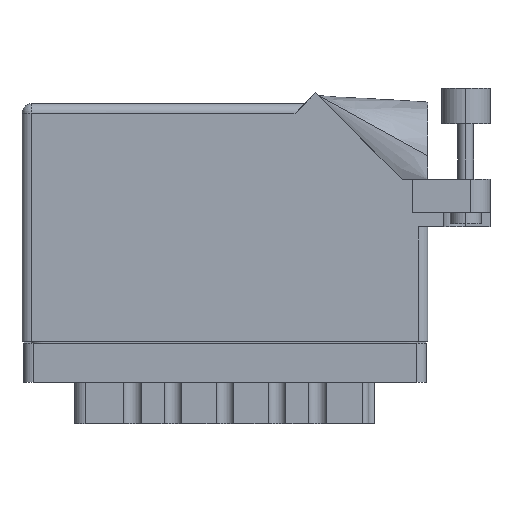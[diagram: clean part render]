
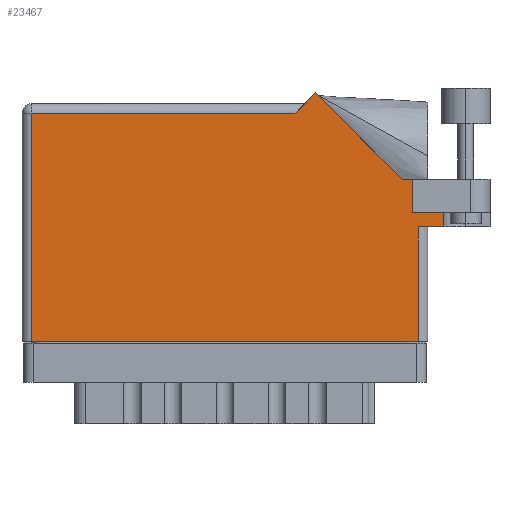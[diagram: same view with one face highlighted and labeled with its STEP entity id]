
A CAD part, front view. The second image highlights one B-rep face of the part: STEP entity #23467.
In plain terms, the highlighted face is planar.
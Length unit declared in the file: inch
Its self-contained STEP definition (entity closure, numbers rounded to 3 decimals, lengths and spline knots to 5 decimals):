
#721 = ORIENTED_EDGE ( 'NONE', *, *, #10785, .T. ) ;
#1046 = CARTESIAN_POINT ( 'NONE',  ( 1.88971, 1.60071, 0. ) ) ;
#1499 = ORIENTED_EDGE ( 'NONE', *, *, #35282, .T. ) ;
#1705 = VERTEX_POINT ( 'NONE', #36975 ) ;
#2884 = DIRECTION ( 'NONE',  ( -0.707, -0.707, 0. ) ) ;
#3130 = VERTEX_POINT ( 'NONE', #36191 ) ;
#4449 = FACE_OUTER_BOUND ( 'NONE', #15342, .T. ) ;
#4676 = ORIENTED_EDGE ( 'NONE', *, *, #24609, .T. ) ;
#5440 = VECTOR ( 'NONE', #20212, 39.37008 ) ;
#6740 = CARTESIAN_POINT ( 'NONE',  ( 1.819, 1.53, 0. ) ) ;
#6857 = VECTOR ( 'NONE', #27558, 39.37008 ) ;
#8744 = LINE ( 'NONE', #10855, #18509 ) ;
#10021 = EDGE_CURVE ( 'NONE', #30598, #53481, #17926, .T. ) ;
#10695 = ORIENTED_EDGE ( 'NONE', *, *, #10021, .F. ) ;
#10785 = EDGE_CURVE ( 'NONE', #21919, #14228, #8744, .T. ) ;
#10855 = CARTESIAN_POINT ( 'NONE',  ( 2.612, 0.737, 0. ) ) ;
#11718 = EDGE_CURVE ( 'NONE', #53481, #14228, #48472, .T. ) ;
#12392 = CARTESIAN_POINT ( 'NONE',  ( 2.512, 0.831, 0. ) ) ;
#13462 = EDGE_CURVE ( 'NONE', #20100, #3130, #17630, .T. ) ;
#13913 = VERTEX_POINT ( 'NONE', #35406 ) ;
#14141 = CARTESIAN_POINT ( 'NONE',  ( 0.062, 0., 0. ) ) ;
#14228 = VERTEX_POINT ( 'NONE', #30231 ) ;
#14478 = AXIS2_PLACEMENT_3D ( 'NONE', #49398, #36578, #32543 ) ;
#15342 = EDGE_LOOP ( 'NONE', ( #4676, #23969, #721, #19280, #10695, #16100, #18601, #21713, #24419, #1499, #52973 ) ) ;
#16100 = ORIENTED_EDGE ( 'NONE', *, *, #40701, .T. ) ;
#16391 = DIRECTION ( 'NONE',  ( -1., 0., 0. ) ) ;
#17299 = CARTESIAN_POINT ( 'NONE',  ( 2.512, 0.831, 0. ) ) ;
#17630 = LINE ( 'NONE', #24145, #35914 ) ;
#17926 = LINE ( 'NONE', #32101, #6857 ) ;
#18509 = VECTOR ( 'NONE', #19446, 39.37008 ) ;
#18561 = VERTEX_POINT ( 'NONE', #14141 ) ;
#18601 = ORIENTED_EDGE ( 'NONE', *, *, #13462, .T. ) ;
#19280 = ORIENTED_EDGE ( 'NONE', *, *, #11718, .F. ) ;
#19446 = DIRECTION ( 'NONE',  ( 1., 0., 0. ) ) ;
#20100 = VERTEX_POINT ( 'NONE', #46377 ) ;
#20212 = DIRECTION ( 'NONE',  ( -0.707, 0.707, 0. ) ) ;
#21713 = ORIENTED_EDGE ( 'NONE', *, *, #42546, .T. ) ;
#21919 = VERTEX_POINT ( 'NONE', #28156 ) ;
#23467 = ADVANCED_FACE ( 'NONE', ( #4449 ), #49220, .F. ) ;
#23969 = ORIENTED_EDGE ( 'NONE', *, *, #43706, .T. ) ;
#24145 = CARTESIAN_POINT ( 'NONE',  ( 3.012, 1.044, 0. ) ) ;
#24419 = ORIENTED_EDGE ( 'NONE', *, *, #42443, .T. ) ;
#24609 = EDGE_CURVE ( 'NONE', #18561, #50068, #49246, .T. ) ;
#25543 = VECTOR ( 'NONE', #50282, 39.37008 ) ;
#26360 = VECTOR ( 'NONE', #33518, 39.37008 ) ;
#26811 = LINE ( 'NONE', #45448, #25543 ) ;
#27558 = DIRECTION ( 'NONE',  ( 1., 0., 0. ) ) ;
#28145 = DIRECTION ( 'NONE',  ( -1., 0., 0. ) ) ;
#28156 = CARTESIAN_POINT ( 'NONE',  ( 2.55, 0.737, 0. ) ) ;
#30231 = CARTESIAN_POINT ( 'NONE',  ( 2.7135, 0.737, 0. ) ) ;
#30491 = VECTOR ( 'NONE', #37020, 39.37008 ) ;
#30598 = VERTEX_POINT ( 'NONE', #17299 ) ;
#31955 = DIRECTION ( 'NONE',  ( 0., -1., 0. ) ) ;
#32101 = CARTESIAN_POINT ( 'NONE',  ( 2.512, 0.831, 0. ) ) ;
#32543 = DIRECTION ( 'NONE',  ( -1., 0., 0. ) ) ;
#33518 = DIRECTION ( 'NONE',  ( 0., -1., 0. ) ) ;
#33697 = CARTESIAN_POINT ( 'NONE',  ( 0., 1.468, 0. ) ) ;
#35005 = VECTOR ( 'NONE', #53698, 39.37008 ) ;
#35282 = EDGE_CURVE ( 'NONE', #13913, #1705, #47054, .T. ) ;
#35406 = CARTESIAN_POINT ( 'NONE',  ( 1.757, 1.468, 0. ) ) ;
#35914 = VECTOR ( 'NONE', #28145, 39.37008 ) ;
#36055 = VECTOR ( 'NONE', #16391, 39.37008 ) ;
#36059 = VECTOR ( 'NONE', #2884, 39.37008 ) ;
#36191 = CARTESIAN_POINT ( 'NONE',  ( 2.44642, 1.044, 0. ) ) ;
#36578 = DIRECTION ( 'NONE',  ( 0., 0., -1. ) ) ;
#36887 = VECTOR ( 'NONE', #31955, 39.37008 ) ;
#36975 = CARTESIAN_POINT ( 'NONE',  ( 0.062, 1.468, 0. ) ) ;
#37020 = DIRECTION ( 'NONE',  ( 0., 1., 0. ) ) ;
#37540 = CARTESIAN_POINT ( 'NONE',  ( 2.7135, 1.16177, 0. ) ) ;
#38149 = VERTEX_POINT ( 'NONE', #1046 ) ;
#40701 = EDGE_CURVE ( 'NONE', #30598, #20100, #44186, .T. ) ;
#41452 = CARTESIAN_POINT ( 'NONE',  ( 2.55, 0., 0. ) ) ;
#42443 = EDGE_CURVE ( 'NONE', #38149, #13913, #48414, .T. ) ;
#42546 = EDGE_CURVE ( 'NONE', #3130, #38149, #45882, .T. ) ;
#43033 = CARTESIAN_POINT ( 'NONE',  ( 2.7135, 0.831, 0. ) ) ;
#43706 = EDGE_CURVE ( 'NONE', #50068, #21919, #26811, .T. ) ;
#44186 = LINE ( 'NONE', #12392, #30491 ) ;
#45198 = CARTESIAN_POINT ( 'NONE',  ( 0., 0., 0. ) ) ;
#45448 = CARTESIAN_POINT ( 'NONE',  ( 2.55, 0.737, 0. ) ) ;
#45500 = CARTESIAN_POINT ( 'NONE',  ( 2.44642, 1.044, 0. ) ) ;
#45882 = LINE ( 'NONE', #45500, #5440 ) ;
#46377 = CARTESIAN_POINT ( 'NONE',  ( 2.512, 1.044, 0. ) ) ;
#47054 = LINE ( 'NONE', #33697, #36055 ) ;
#48387 = EDGE_CURVE ( 'NONE', #1705, #18561, #50452, .T. ) ;
#48414 = LINE ( 'NONE', #6740, #36059 ) ;
#48472 = LINE ( 'NONE', #37540, #26360 ) ;
#49220 = PLANE ( 'NONE',  #14478 ) ;
#49246 = LINE ( 'NONE', #45198, #35005 ) ;
#49398 = CARTESIAN_POINT ( 'NONE',  ( 0., 1.53, 0. ) ) ;
#50068 = VERTEX_POINT ( 'NONE', #41452 ) ;
#50282 = DIRECTION ( 'NONE',  ( 0., 1., 0. ) ) ;
#50452 = LINE ( 'NONE', #53207, #36887 ) ;
#52973 = ORIENTED_EDGE ( 'NONE', *, *, #48387, .T. ) ;
#53207 = CARTESIAN_POINT ( 'NONE',  ( 0.062, 0., 0. ) ) ;
#53481 = VERTEX_POINT ( 'NONE', #43033 ) ;
#53698 = DIRECTION ( 'NONE',  ( 1., 0., 0. ) ) ;
